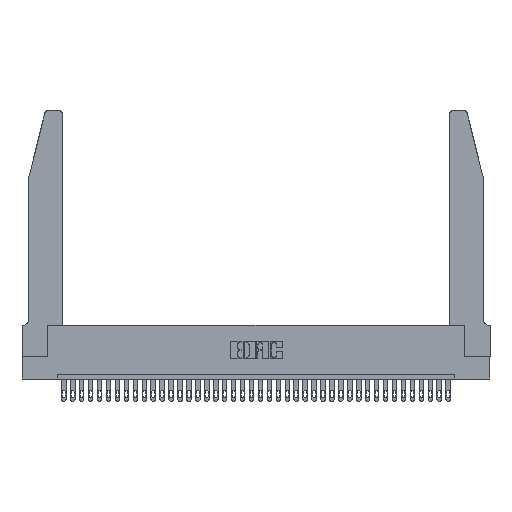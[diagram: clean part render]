
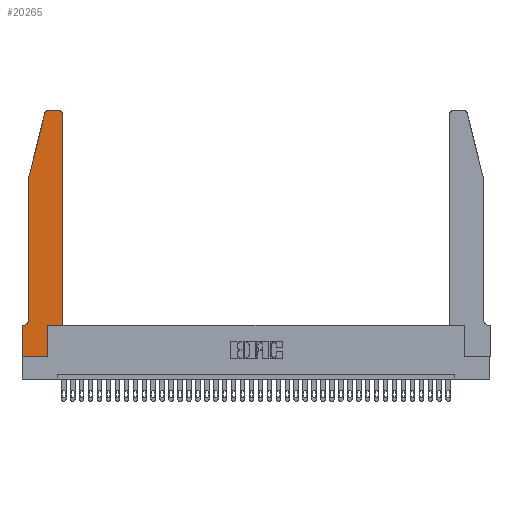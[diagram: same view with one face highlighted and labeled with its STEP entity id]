
A CAD part, top view. The second image highlights one B-rep face of the part: STEP entity #20265.
In plain terms, the highlighted planar face has unit normal (0, 0, 1).
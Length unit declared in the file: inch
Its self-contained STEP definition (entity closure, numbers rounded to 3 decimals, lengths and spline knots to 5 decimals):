
#209 = CARTESIAN_POINT ( 'NONE',  ( 0.0755, 0.35, 0.37 ) ) ;
#1342 = CARTESIAN_POINT ( 'NONE',  ( 0.4505, 0.35, 0.37 ) ) ;
#1711 = EDGE_LOOP ( 'NONE', ( #16465, #17793, #16059, #33931, #14583, #13746, #34080, #28322, #24379, #25672, #8215, #9153 ) ) ;
#1931 = DIRECTION ( 'NONE',  ( 0., 0., 1. ) ) ;
#2445 = EDGE_CURVE ( 'NONE', #16035, #9840, #14686, .T. ) ;
#2767 = DIRECTION ( 'NONE',  ( -0.239, -0.971, 0. ) ) ;
#2903 = DIRECTION ( 'NONE',  ( 1., 0., 0. ) ) ;
#2978 = EDGE_CURVE ( 'NONE', #16483, #17352, #17676, .T. ) ;
#3020 = CARTESIAN_POINT ( 'NONE',  ( 0., 0., 0.37 ) ) ;
#3114 = DIRECTION ( 'NONE',  ( -1., 0., 0. ) ) ;
#3293 = VERTEX_POINT ( 'NONE', #20074 ) ;
#3380 = DIRECTION ( 'NONE',  ( 1., 0., 0. ) ) ;
#3713 = VECTOR ( 'NONE', #2767, 39.37008 ) ;
#3753 = VECTOR ( 'NONE', #9047, 39.37008 ) ;
#3814 = CARTESIAN_POINT ( 'NONE',  ( 0.0755, 2., 0.37 ) ) ;
#4021 = VECTOR ( 'NONE', #2903, 39.37008 ) ;
#4323 = DIRECTION ( 'NONE',  ( -1., 0., 0. ) ) ;
#4514 = EDGE_CURVE ( 'NONE', #21026, #34141, #15733, .T. ) ;
#5422 = CARTESIAN_POINT ( 'NONE',  ( 0.25487, 2.72718, 0.37 ) ) ;
#5660 = DIRECTION ( 'NONE',  ( 0., 0., -1. ) ) ;
#6104 = DIRECTION ( 'NONE',  ( -1., 0., 0. ) ) ;
#6150 = CARTESIAN_POINT ( 'NONE',  ( 0.2865, 0.35, 0.37 ) ) ;
#6249 = EDGE_CURVE ( 'NONE', #17352, #8840, #16078, .T. ) ;
#6478 = FACE_OUTER_BOUND ( 'NONE', #1711, .T. ) ;
#6994 = CARTESIAN_POINT ( 'NONE',  ( 0.4205, 2.72, 0.37 ) ) ;
#7095 = CARTESIAN_POINT ( 'NONE',  ( 0.4505, 0.35, 0.37 ) ) ;
#7555 = DIRECTION ( 'NONE',  ( 0., 0., 1. ) ) ;
#7938 = DIRECTION ( 'NONE',  ( 0., -1., 0. ) ) ;
#8215 = ORIENTED_EDGE ( 'NONE', *, *, #2978, .T. ) ;
#8583 = LINE ( 'NONE', #9859, #11729 ) ;
#8840 = VERTEX_POINT ( 'NONE', #34674 ) ;
#9045 = AXIS2_PLACEMENT_3D ( 'NONE', #15741, #5660, #6104 ) ;
#9047 = DIRECTION ( 'NONE',  ( 0., 1., 0. ) ) ;
#9153 = ORIENTED_EDGE ( 'NONE', *, *, #6249, .T. ) ;
#9215 = LINE ( 'NONE', #209, #35578 ) ;
#9840 = VERTEX_POINT ( 'NONE', #5422 ) ;
#9859 = CARTESIAN_POINT ( 'NONE',  ( 0.2605, 2.75, 0.37 ) ) ;
#10462 = VECTOR ( 'NONE', #18818, 39.37008 ) ;
#10658 = CARTESIAN_POINT ( 'NONE',  ( 0.4505, 2.72, 0.37 ) ) ;
#11729 = VECTOR ( 'NONE', #4323, 39.37008 ) ;
#11842 = CARTESIAN_POINT ( 'NONE',  ( 0.284, 2.72, 0.37 ) ) ;
#12339 = EDGE_CURVE ( 'NONE', #8840, #16035, #8583, .T. ) ;
#13746 = ORIENTED_EDGE ( 'NONE', *, *, #33816, .T. ) ;
#14155 = AXIS2_PLACEMENT_3D ( 'NONE', #24806, #7555, #26709 ) ;
#14426 = VECTOR ( 'NONE', #23984, 39.37008 ) ;
#14583 = ORIENTED_EDGE ( 'NONE', *, *, #4514, .T. ) ;
#14686 = CIRCLE ( 'NONE', #21062, 0.03 ) ;
#14980 = CARTESIAN_POINT ( 'NONE',  ( 0.0755, 0.42, 0.37 ) ) ;
#15107 = CARTESIAN_POINT ( 'NONE',  ( 0.284, 2.75, 0.37 ) ) ;
#15273 = EDGE_CURVE ( 'NONE', #17090, #16483, #20538, .T. ) ;
#15419 = DIRECTION ( 'NONE',  ( 0., 0., 1. ) ) ;
#15733 = CIRCLE ( 'NONE', #9045, 0.07 ) ;
#15741 = CARTESIAN_POINT ( 'NONE',  ( 0.0055, 0.42, 0.37 ) ) ;
#15924 = DIRECTION ( 'NONE',  ( 1., 0., 0. ) ) ;
#16019 = VERTEX_POINT ( 'NONE', #32095 ) ;
#16035 = VERTEX_POINT ( 'NONE', #15107 ) ;
#16059 = ORIENTED_EDGE ( 'NONE', *, *, #35287, .T. ) ;
#16078 = CIRCLE ( 'NONE', #17275, 0.03 ) ;
#16325 = VERTEX_POINT ( 'NONE', #36394 ) ;
#16465 = ORIENTED_EDGE ( 'NONE', *, *, #12339, .T. ) ;
#16483 = VERTEX_POINT ( 'NONE', #26517 ) ;
#16618 = LINE ( 'NONE', #3020, #4021 ) ;
#16957 = VECTOR ( 'NONE', #35874, 39.37008 ) ;
#17090 = VERTEX_POINT ( 'NONE', #18374 ) ;
#17275 = AXIS2_PLACEMENT_3D ( 'NONE', #6994, #15419, #15924 ) ;
#17352 = VERTEX_POINT ( 'NONE', #10658 ) ;
#17485 = LINE ( 'NONE', #6150, #3753 ) ;
#17676 = LINE ( 'NONE', #7095, #10462 ) ;
#17793 = ORIENTED_EDGE ( 'NONE', *, *, #2445, .T. ) ;
#18374 = CARTESIAN_POINT ( 'NONE',  ( 0.2865, 0.35, 0.37 ) ) ;
#18818 = DIRECTION ( 'NONE',  ( 0., 1., 0. ) ) ;
#20074 = CARTESIAN_POINT ( 'NONE',  ( 0., 0.35, 0.37 ) ) ;
#20265 = ADVANCED_FACE ( 'NONE', ( #6478 ), #36502, .T. ) ;
#20538 = LINE ( 'NONE', #1342, #16957 ) ;
#20841 = VECTOR ( 'NONE', #7938, 39.37008 ) ;
#21026 = VERTEX_POINT ( 'NONE', #14980 ) ;
#21062 = AXIS2_PLACEMENT_3D ( 'NONE', #11842, #1931, #3380 ) ;
#21985 = VERTEX_POINT ( 'NONE', #33725 ) ;
#22208 = LINE ( 'NONE', #33935, #20841 ) ;
#23658 = EDGE_CURVE ( 'NONE', #21985, #16325, #16618, .T. ) ;
#23984 = DIRECTION ( 'NONE',  ( 0., -1., 0. ) ) ;
#24367 = LINE ( 'NONE', #3814, #14426 ) ;
#24379 = ORIENTED_EDGE ( 'NONE', *, *, #34731, .T. ) ;
#24806 = CARTESIAN_POINT ( 'NONE',  ( 0., 0.35, 0.37 ) ) ;
#25672 = ORIENTED_EDGE ( 'NONE', *, *, #15273, .T. ) ;
#25780 = LINE ( 'NONE', #31552, #3713 ) ;
#26517 = CARTESIAN_POINT ( 'NONE',  ( 0.4505, 0.35, 0.37 ) ) ;
#26709 = DIRECTION ( 'NONE',  ( 1., 0., 0. ) ) ;
#28049 = EDGE_CURVE ( 'NONE', #3293, #21985, #22208, .T. ) ;
#28322 = ORIENTED_EDGE ( 'NONE', *, *, #23658, .T. ) ;
#30207 = CARTESIAN_POINT ( 'NONE',  ( 0.0055, 0.35, 0.37 ) ) ;
#31552 = CARTESIAN_POINT ( 'NONE',  ( 0.0755, 2., 0.37 ) ) ;
#32095 = CARTESIAN_POINT ( 'NONE',  ( 0.0755, 2., 0.37 ) ) ;
#33725 = CARTESIAN_POINT ( 'NONE',  ( 0., 0., 0.37 ) ) ;
#33816 = EDGE_CURVE ( 'NONE', #34141, #3293, #9215, .T. ) ;
#33931 = ORIENTED_EDGE ( 'NONE', *, *, #36241, .T. ) ;
#33935 = CARTESIAN_POINT ( 'NONE',  ( 0., 0., 0.37 ) ) ;
#34080 = ORIENTED_EDGE ( 'NONE', *, *, #28049, .T. ) ;
#34141 = VERTEX_POINT ( 'NONE', #30207 ) ;
#34674 = CARTESIAN_POINT ( 'NONE',  ( 0.4205, 2.75, 0.37 ) ) ;
#34731 = EDGE_CURVE ( 'NONE', #16325, #17090, #17485, .T. ) ;
#35287 = EDGE_CURVE ( 'NONE', #9840, #16019, #25780, .T. ) ;
#35578 = VECTOR ( 'NONE', #3114, 39.37008 ) ;
#35874 = DIRECTION ( 'NONE',  ( 1., 0., 0. ) ) ;
#36241 = EDGE_CURVE ( 'NONE', #16019, #21026, #24367, .T. ) ;
#36394 = CARTESIAN_POINT ( 'NONE',  ( 0.2865, 0., 0.37 ) ) ;
#36502 = PLANE ( 'NONE',  #14155 ) ;
